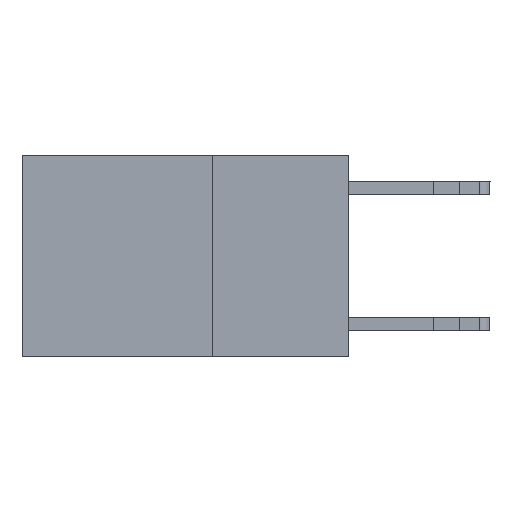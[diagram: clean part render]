
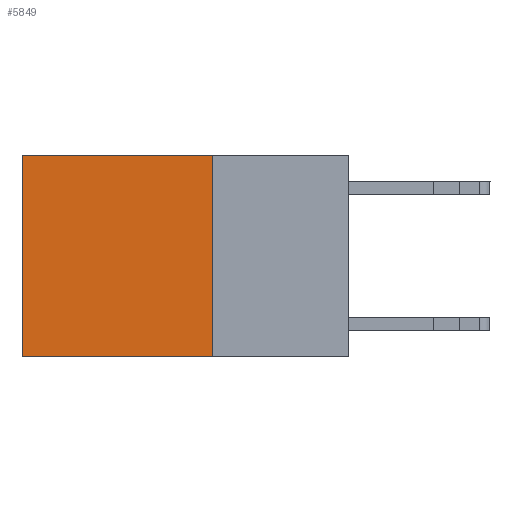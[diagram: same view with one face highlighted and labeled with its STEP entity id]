
A CAD part, left-side view. The second image highlights one B-rep face of the part: STEP entity #5849.
In plain terms, the highlighted planar face has unit normal (-1, 0, 0).
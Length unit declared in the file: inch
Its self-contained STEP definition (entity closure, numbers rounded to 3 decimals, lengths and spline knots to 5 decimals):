
#28 = CARTESIAN_POINT ( 'NONE',  ( 0.2625, 0.25, 0. ) ) ;
#151 = CARTESIAN_POINT ( 'NONE',  ( 0.2625, 0.6, 0. ) ) ;
#152 = ORIENTED_EDGE ( 'NONE', *, *, #6344, .F. ) ;
#317 = VECTOR ( 'NONE', #7139, 39.37008 ) ;
#328 = DIRECTION ( 'NONE',  ( 0., 1., 0. ) ) ;
#1970 = DIRECTION ( 'NONE',  ( 0., 0., -1. ) ) ;
#2028 = VERTEX_POINT ( 'NONE', #3444 ) ;
#3177 = DIRECTION ( 'NONE',  ( 0., 0., -1. ) ) ;
#3444 = CARTESIAN_POINT ( 'NONE',  ( 0.2625, 0.25, -0.37 ) ) ;
#3905 = ORIENTED_EDGE ( 'NONE', *, *, #12638, .T. ) ;
#4228 = LINE ( 'NONE', #5440, #7211 ) ;
#4392 = AXIS2_PLACEMENT_3D ( 'NONE', #28, #4947, #1970 ) ;
#4580 = EDGE_LOOP ( 'NONE', ( #3905, #152, #12069, #12876 ) ) ;
#4924 = VECTOR ( 'NONE', #3177, 39.37008 ) ;
#4947 = DIRECTION ( 'NONE',  ( 1., 0., 0. ) ) ;
#5440 = CARTESIAN_POINT ( 'NONE',  ( 0.2625, 0.25, 0. ) ) ;
#5849 = ADVANCED_FACE ( 'NONE', ( #11145 ), #13258, .F. ) ;
#6046 = VERTEX_POINT ( 'NONE', #151 ) ;
#6344 = EDGE_CURVE ( 'NONE', #2028, #8717, #11591, .T. ) ;
#6807 = CARTESIAN_POINT ( 'NONE',  ( 0.2625, 0.6, -0.37 ) ) ;
#7139 = DIRECTION ( 'NONE',  ( 0., 1., 0. ) ) ;
#7211 = VECTOR ( 'NONE', #7352, 39.37008 ) ;
#7232 = EDGE_CURVE ( 'NONE', #10795, #6046, #8202, .T. ) ;
#7352 = DIRECTION ( 'NONE',  ( 0., 0., -1. ) ) ;
#7433 = VECTOR ( 'NONE', #328, 39.37008 ) ;
#8107 = EDGE_CURVE ( 'NONE', #10795, #2028, #4228, .T. ) ;
#8124 = CARTESIAN_POINT ( 'NONE',  ( 0.2625, 0.25, 0. ) ) ;
#8202 = LINE ( 'NONE', #8124, #317 ) ;
#8433 = LINE ( 'NONE', #11349, #4924 ) ;
#8599 = CARTESIAN_POINT ( 'NONE',  ( 0.2625, 0.25, 0. ) ) ;
#8717 = VERTEX_POINT ( 'NONE', #6807 ) ;
#10625 = CARTESIAN_POINT ( 'NONE',  ( 0.2625, 0.25, -0.37 ) ) ;
#10795 = VERTEX_POINT ( 'NONE', #8599 ) ;
#11145 = FACE_OUTER_BOUND ( 'NONE', #4580, .T. ) ;
#11349 = CARTESIAN_POINT ( 'NONE',  ( 0.2625, 0.6, 0. ) ) ;
#11591 = LINE ( 'NONE', #10625, #7433 ) ;
#12069 = ORIENTED_EDGE ( 'NONE', *, *, #8107, .F. ) ;
#12638 = EDGE_CURVE ( 'NONE', #6046, #8717, #8433, .T. ) ;
#12876 = ORIENTED_EDGE ( 'NONE', *, *, #7232, .T. ) ;
#13258 = PLANE ( 'NONE',  #4392 ) ;
